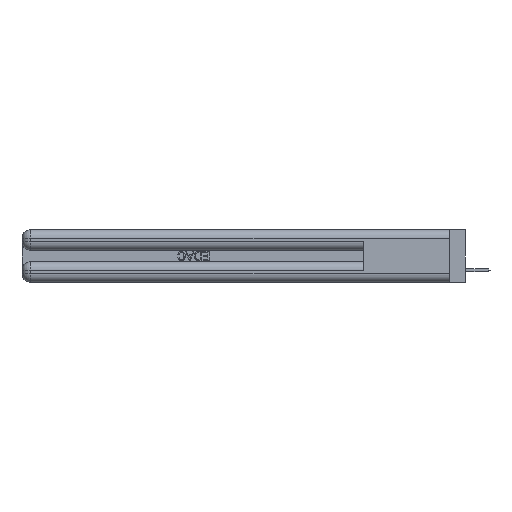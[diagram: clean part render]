
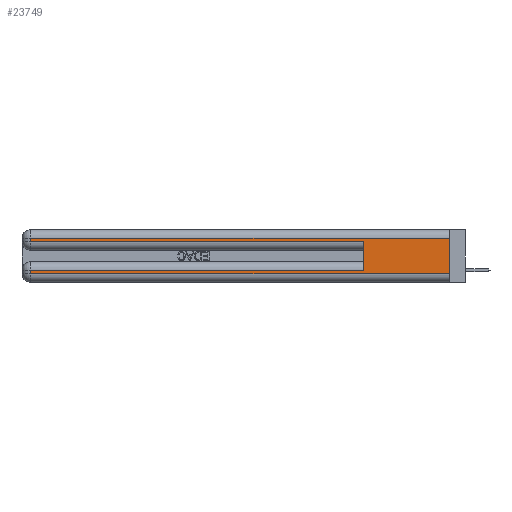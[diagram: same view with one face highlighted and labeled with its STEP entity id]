
A CAD part, left-side view. The second image highlights one B-rep face of the part: STEP entity #23749.
In plain terms, the highlighted planar face has unit normal (-1, 0, 0).
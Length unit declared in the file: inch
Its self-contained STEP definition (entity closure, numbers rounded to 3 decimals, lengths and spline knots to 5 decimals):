
#313 = VECTOR ( 'NONE', #6062, 39.37008 ) ;
#587 = VERTEX_POINT ( 'NONE', #7773 ) ;
#3056 = VECTOR ( 'NONE', #13534, 39.37008 ) ;
#3879 = LINE ( 'NONE', #32753, #37850 ) ;
#3888 = EDGE_CURVE ( 'NONE', #12862, #32942, #22568, .T. ) ;
#4384 = CARTESIAN_POINT ( 'NONE',  ( 0., 0., 0.085 ) ) ;
#6004 = CARTESIAN_POINT ( 'NONE',  ( 0., 2.94, 0.285 ) ) ;
#6062 = DIRECTION ( 'NONE',  ( 0., 0., -1. ) ) ;
#6266 = DIRECTION ( 'NONE',  ( 0., -1., 0. ) ) ;
#7147 = VECTOR ( 'NONE', #7979, 39.37008 ) ;
#7773 = CARTESIAN_POINT ( 'NONE',  ( 0., 2.94, 0.31 ) ) ;
#7979 = DIRECTION ( 'NONE',  ( 0., 1., 0. ) ) ;
#8215 = CARTESIAN_POINT ( 'NONE',  ( 0., 2.94, 0.37 ) ) ;
#8673 = VECTOR ( 'NONE', #21858, 39.37008 ) ;
#9804 = EDGE_CURVE ( 'NONE', #40797, #29270, #3879, .T. ) ;
#11651 = CARTESIAN_POINT ( 'NONE',  ( 0., 0.6, 0.145 ) ) ;
#11874 = VECTOR ( 'NONE', #27338, 39.37008 ) ;
#12677 = FACE_OUTER_BOUND ( 'NONE', #15761, .T. ) ;
#12862 = VERTEX_POINT ( 'NONE', #38244 ) ;
#13534 = DIRECTION ( 'NONE',  ( 0., -1., 0. ) ) ;
#13727 = CARTESIAN_POINT ( 'NONE',  ( 0., 0., 0.37 ) ) ;
#14679 = CARTESIAN_POINT ( 'NONE',  ( 0., 0., 0.31 ) ) ;
#14925 = LINE ( 'NONE', #4384, #11874 ) ;
#15761 = EDGE_LOOP ( 'NONE', ( #19912, #21335, #21166, #23264, #42224, #31517, #42333, #36473 ) ) ;
#16645 = EDGE_CURVE ( 'NONE', #30585, #34386, #32305, .T. ) ;
#17601 = CARTESIAN_POINT ( 'NONE',  ( 0., 0., 0.31 ) ) ;
#18546 = LINE ( 'NONE', #17601, #7147 ) ;
#18797 = EDGE_CURVE ( 'NONE', #38077, #32942, #32028, .T. ) ;
#18928 = CARTESIAN_POINT ( 'NONE',  ( 0., 2.94, 0.085 ) ) ;
#19912 = ORIENTED_EDGE ( 'NONE', *, *, #9804, .F. ) ;
#20390 = EDGE_CURVE ( 'NONE', #12862, #30585, #14925, .T. ) ;
#21163 = AXIS2_PLACEMENT_3D ( 'NONE', #13727, #36682, #39983 ) ;
#21166 = ORIENTED_EDGE ( 'NONE', *, *, #31366, .T. ) ;
#21335 = ORIENTED_EDGE ( 'NONE', *, *, #28695, .T. ) ;
#21666 = CARTESIAN_POINT ( 'NONE',  ( 0., 0., 0.06 ) ) ;
#21858 = DIRECTION ( 'NONE',  ( 0., 0., 1. ) ) ;
#22291 = VECTOR ( 'NONE', #6266, 39.37008 ) ;
#22447 = CARTESIAN_POINT ( 'NONE',  ( 0., 0.6, 0.285 ) ) ;
#22568 = LINE ( 'NONE', #11651, #8673 ) ;
#23264 = ORIENTED_EDGE ( 'NONE', *, *, #18797, .T. ) ;
#23749 = ADVANCED_FACE ( 'NONE', ( #12677 ), #33359, .F. ) ;
#24045 = LINE ( 'NONE', #36921, #3056 ) ;
#24520 = LINE ( 'NONE', #35509, #313 ) ;
#27338 = DIRECTION ( 'NONE',  ( 0., 1., 0. ) ) ;
#27697 = DIRECTION ( 'NONE',  ( 0., 0., -1. ) ) ;
#28695 = EDGE_CURVE ( 'NONE', #40797, #587, #18546, .T. ) ;
#29270 = VERTEX_POINT ( 'NONE', #21666 ) ;
#30585 = VERTEX_POINT ( 'NONE', #18928 ) ;
#31366 = EDGE_CURVE ( 'NONE', #587, #38077, #24520, .T. ) ;
#31517 = ORIENTED_EDGE ( 'NONE', *, *, #20390, .T. ) ;
#32028 = LINE ( 'NONE', #35727, #22291 ) ;
#32305 = LINE ( 'NONE', #8215, #38971 ) ;
#32753 = CARTESIAN_POINT ( 'NONE',  ( 0., 0., 0.37 ) ) ;
#32942 = VERTEX_POINT ( 'NONE', #22447 ) ;
#33359 = PLANE ( 'NONE',  #21163 ) ;
#34386 = VERTEX_POINT ( 'NONE', #40465 ) ;
#35509 = CARTESIAN_POINT ( 'NONE',  ( 0., 2.94, 0.37 ) ) ;
#35727 = CARTESIAN_POINT ( 'NONE',  ( 0., 0., 0.285 ) ) ;
#35813 = DIRECTION ( 'NONE',  ( 0., 0., -1. ) ) ;
#36473 = ORIENTED_EDGE ( 'NONE', *, *, #38509, .T. ) ;
#36682 = DIRECTION ( 'NONE',  ( 1., 0., 0. ) ) ;
#36921 = CARTESIAN_POINT ( 'NONE',  ( 0., 0., 0.06 ) ) ;
#37850 = VECTOR ( 'NONE', #35813, 39.37008 ) ;
#38077 = VERTEX_POINT ( 'NONE', #6004 ) ;
#38244 = CARTESIAN_POINT ( 'NONE',  ( 0., 0.6, 0.085 ) ) ;
#38509 = EDGE_CURVE ( 'NONE', #34386, #29270, #24045, .T. ) ;
#38971 = VECTOR ( 'NONE', #27697, 39.37008 ) ;
#39983 = DIRECTION ( 'NONE',  ( 0., 0., -1. ) ) ;
#40465 = CARTESIAN_POINT ( 'NONE',  ( 0., 2.94, 0.06 ) ) ;
#40797 = VERTEX_POINT ( 'NONE', #14679 ) ;
#42224 = ORIENTED_EDGE ( 'NONE', *, *, #3888, .F. ) ;
#42333 = ORIENTED_EDGE ( 'NONE', *, *, #16645, .T. ) ;
